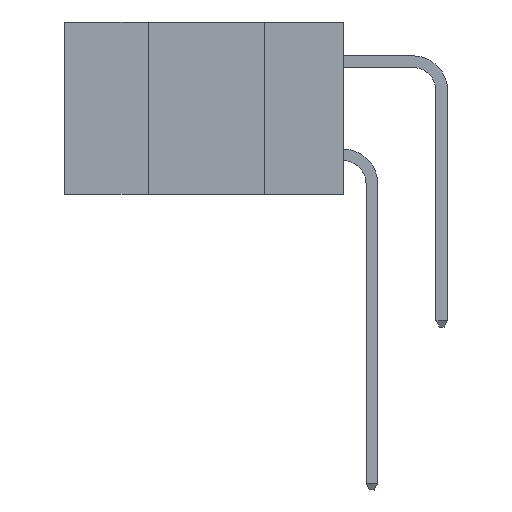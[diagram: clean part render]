
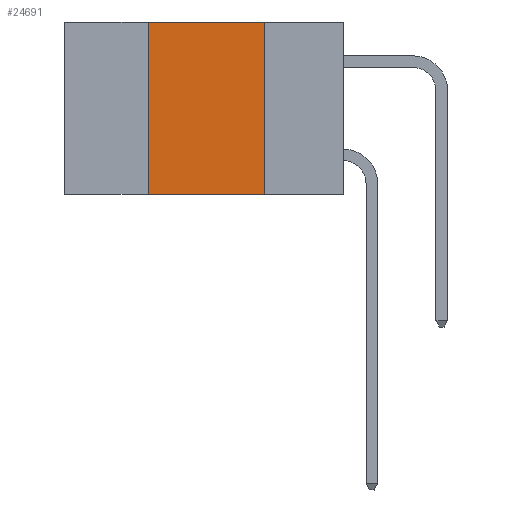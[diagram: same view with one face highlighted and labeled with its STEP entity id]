
A CAD part, left-side view. The second image highlights one B-rep face of the part: STEP entity #24691.
In plain terms, the highlighted planar face has unit normal (-1, 0, 0).
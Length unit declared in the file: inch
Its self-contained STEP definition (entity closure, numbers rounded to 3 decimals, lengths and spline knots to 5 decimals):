
#773 = AXIS2_PLACEMENT_3D ( 'NONE', #4586, #9489, #26327 ) ;
#2691 = VERTEX_POINT ( 'NONE', #20591 ) ;
#2832 = EDGE_CURVE ( 'NONE', #10713, #23588, #5082, .T. ) ;
#3195 = VERTEX_POINT ( 'NONE', #7093 ) ;
#4586 = CARTESIAN_POINT ( 'NONE',  ( 0., 0.6, 0. ) ) ;
#4751 = DIRECTION ( 'NONE',  ( 0., -1., 0. ) ) ;
#5082 = LINE ( 'NONE', #7971, #23565 ) ;
#5167 = LINE ( 'NONE', #14434, #17184 ) ;
#6830 = LINE ( 'NONE', #27591, #12361 ) ;
#7093 = CARTESIAN_POINT ( 'NONE',  ( 0., 0.17, 0. ) ) ;
#7157 = EDGE_LOOP ( 'NONE', ( #10763, #17134, #12224, #25125 ) ) ;
#7971 = CARTESIAN_POINT ( 'NONE',  ( 0., 0.6, -0.37 ) ) ;
#9407 = EDGE_CURVE ( 'NONE', #10713, #2691, #6830, .T. ) ;
#9489 = DIRECTION ( 'NONE',  ( 1., 0., 0. ) ) ;
#10713 = VERTEX_POINT ( 'NONE', #22574 ) ;
#10763 = ORIENTED_EDGE ( 'NONE', *, *, #15762, .F. ) ;
#12224 = ORIENTED_EDGE ( 'NONE', *, *, #9407, .F. ) ;
#12361 = VECTOR ( 'NONE', #25167, 39.37008 ) ;
#14434 = CARTESIAN_POINT ( 'NONE',  ( 0., 0.17, 0. ) ) ;
#15762 = EDGE_CURVE ( 'NONE', #3195, #23588, #5167, .T. ) ;
#15767 = DIRECTION ( 'NONE',  ( 0., -1., 0. ) ) ;
#16734 = CARTESIAN_POINT ( 'NONE',  ( 0., 0.6, 0. ) ) ;
#17134 = ORIENTED_EDGE ( 'NONE', *, *, #21859, .F. ) ;
#17184 = VECTOR ( 'NONE', #19353, 39.37008 ) ;
#19353 = DIRECTION ( 'NONE',  ( 0., 0., -1. ) ) ;
#19861 = VECTOR ( 'NONE', #4751, 39.37008 ) ;
#20591 = CARTESIAN_POINT ( 'NONE',  ( 0., 0.42, 0. ) ) ;
#20615 = LINE ( 'NONE', #16734, #19861 ) ;
#21859 = EDGE_CURVE ( 'NONE', #2691, #3195, #20615, .T. ) ;
#22574 = CARTESIAN_POINT ( 'NONE',  ( 0., 0.42, -0.37 ) ) ;
#23565 = VECTOR ( 'NONE', #15767, 39.37008 ) ;
#23588 = VERTEX_POINT ( 'NONE', #30383 ) ;
#23849 = FACE_OUTER_BOUND ( 'NONE', #7157, .T. ) ;
#23899 = PLANE ( 'NONE',  #773 ) ;
#24691 = ADVANCED_FACE ( 'NONE', ( #23849 ), #23899, .F. ) ;
#25125 = ORIENTED_EDGE ( 'NONE', *, *, #2832, .T. ) ;
#25167 = DIRECTION ( 'NONE',  ( 0., 0., 1. ) ) ;
#26327 = DIRECTION ( 'NONE',  ( 0., 0., -1. ) ) ;
#27591 = CARTESIAN_POINT ( 'NONE',  ( 0., 0.42, 0. ) ) ;
#30383 = CARTESIAN_POINT ( 'NONE',  ( 0., 0.17, -0.37 ) ) ;
